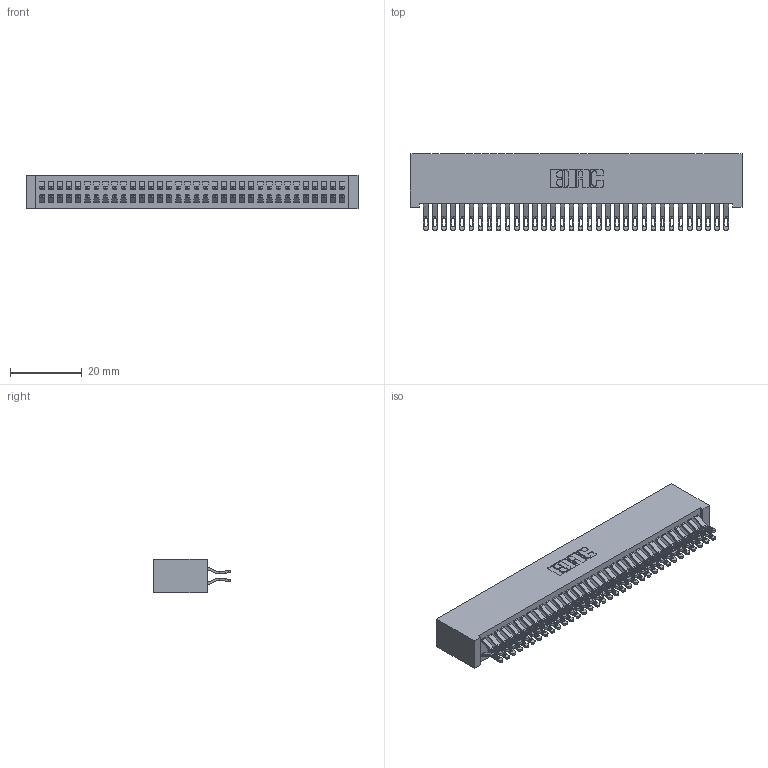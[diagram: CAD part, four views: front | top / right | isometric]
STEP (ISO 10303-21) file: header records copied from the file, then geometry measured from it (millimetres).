
FILE_DESCRIPTION (( 'STEP AP203' ), '1' );
FILE_NAME ('392-068-555-201.STEP', '2018-08-17T22:58:45', ( '' ), ( '' ), 'SwSTEP 2.0', 'SolidWorks 2016', '' );
FILE_SCHEMA (( 'CONFIG_CONTROL_DESIGN' ));
Length unit declared in the file: inch
Products named in the file (3): 392-068-555-201; 342 Part_Lugless; 345-292-001_555 Tail
Assembly tree (69 placements, depth 2):
  392-068-555-201
    342 Part_Lugless
    345-292-001_555 Tail  x68
Bounding box: 92.61 x 21.47 x 9.4 mm (x, y, z)
Volume: 8911.5 mm3; surface area: 15412.7 mm2
Topology: 69 solids, 69 shells, 4046 faces, 12719 edges, 8478 vertices
Faces by surface type: plane 2374, cylinder 1672
Entity records: 22825 total; most frequent: CARTESIAN_POINT 3824, ORIENTED_EDGE 3730, DIRECTION 3245, EDGE_CURVE 1865, VECTOR 1725, LINE 1725, VERTEX_POINT 1242, AXIS2_PLACEMENT_3D 760
